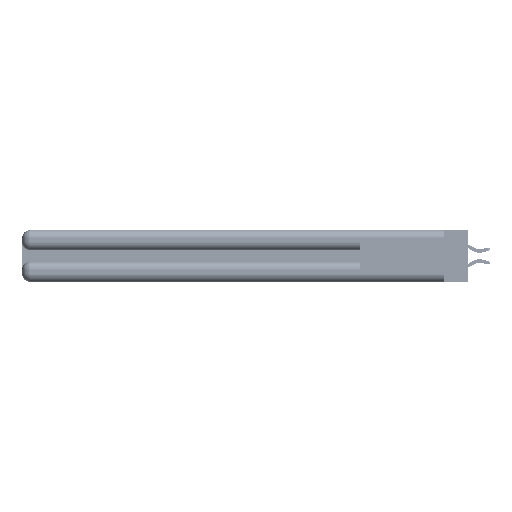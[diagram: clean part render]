
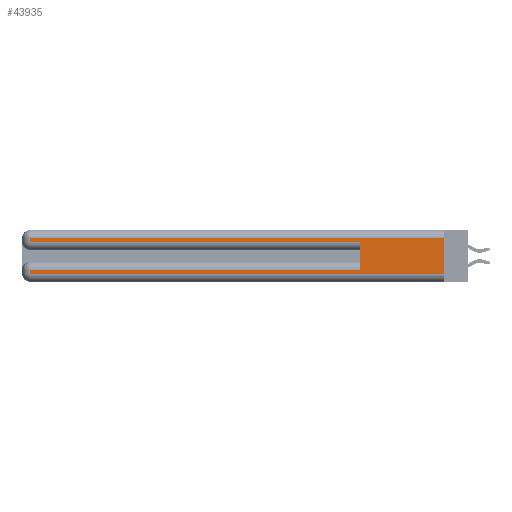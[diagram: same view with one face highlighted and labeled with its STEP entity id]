
A CAD part, left-side view. The second image highlights one B-rep face of the part: STEP entity #43935.
In plain terms, the highlighted planar face has unit normal (-1, 0, 0).
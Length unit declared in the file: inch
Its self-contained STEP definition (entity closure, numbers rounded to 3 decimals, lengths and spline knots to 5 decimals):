
#156 = CARTESIAN_POINT ( 'NONE',  ( 0., 0., 0.37 ) ) ;
#1914 = EDGE_CURVE ( 'NONE', #38945, #14404, #46046, .T. ) ;
#2449 = ORIENTED_EDGE ( 'NONE', *, *, #48243, .T. ) ;
#3163 = VECTOR ( 'NONE', #41741, 39.37008 ) ;
#4113 = EDGE_CURVE ( 'NONE', #38985, #38945, #40312, .T. ) ;
#4177 = DIRECTION ( 'NONE',  ( 0., 0., -1. ) ) ;
#4496 = CARTESIAN_POINT ( 'NONE',  ( 0., 2.94, 0.06 ) ) ;
#4733 = CARTESIAN_POINT ( 'NONE',  ( 0., 0., 0.285 ) ) ;
#7705 = VECTOR ( 'NONE', #36202, 39.37008 ) ;
#8487 = LINE ( 'NONE', #11808, #47719 ) ;
#9057 = EDGE_CURVE ( 'NONE', #34411, #14404, #26335, .T. ) ;
#10881 = DIRECTION ( 'NONE',  ( 0., 0., -1. ) ) ;
#11180 = CARTESIAN_POINT ( 'NONE',  ( 0., 2.94, 0.37 ) ) ;
#11744 = EDGE_CURVE ( 'NONE', #30185, #33494, #34601, .T. ) ;
#11808 = CARTESIAN_POINT ( 'NONE',  ( 0., 0.6, 0.145 ) ) ;
#11882 = ORIENTED_EDGE ( 'NONE', *, *, #9057, .F. ) ;
#12680 = CARTESIAN_POINT ( 'NONE',  ( 0., 2.94, 0.085 ) ) ;
#13272 = CARTESIAN_POINT ( 'NONE',  ( 0., 0., 0.06 ) ) ;
#14369 = CARTESIAN_POINT ( 'NONE',  ( 0., 0., 0.31 ) ) ;
#14404 = VERTEX_POINT ( 'NONE', #14673 ) ;
#14500 = CARTESIAN_POINT ( 'NONE',  ( 0., 2.94, 0.285 ) ) ;
#14673 = CARTESIAN_POINT ( 'NONE',  ( 0., 0., 0.06 ) ) ;
#15150 = DIRECTION ( 'NONE',  ( 0., 0., -1. ) ) ;
#15244 = VECTOR ( 'NONE', #17268, 39.37008 ) ;
#17268 = DIRECTION ( 'NONE',  ( 0., 1., 0. ) ) ;
#18251 = LINE ( 'NONE', #4733, #7705 ) ;
#19418 = EDGE_CURVE ( 'NONE', #33494, #39468, #18251, .T. ) ;
#19722 = CARTESIAN_POINT ( 'NONE',  ( 0., 0.6, 0.085 ) ) ;
#21743 = ORIENTED_EDGE ( 'NONE', *, *, #19418, .T. ) ;
#25411 = ORIENTED_EDGE ( 'NONE', *, *, #4113, .T. ) ;
#26335 = LINE ( 'NONE', #30435, #44681 ) ;
#26481 = VECTOR ( 'NONE', #40627, 39.37008 ) ;
#27783 = DIRECTION ( 'NONE',  ( 1., 0., 0. ) ) ;
#28116 = LINE ( 'NONE', #28885, #15244 ) ;
#28414 = EDGE_LOOP ( 'NONE', ( #11882, #2449, #42818, #21743, #45611, #45478, #25411, #43830 ) ) ;
#28479 = EDGE_CURVE ( 'NONE', #30929, #38985, #28116, .T. ) ;
#28885 = CARTESIAN_POINT ( 'NONE',  ( 0., 0., 0.085 ) ) ;
#30185 = VERTEX_POINT ( 'NONE', #39277 ) ;
#30435 = CARTESIAN_POINT ( 'NONE',  ( 0., 0., 0.37 ) ) ;
#30929 = VERTEX_POINT ( 'NONE', #19722 ) ;
#33494 = VERTEX_POINT ( 'NONE', #14500 ) ;
#34411 = VERTEX_POINT ( 'NONE', #36673 ) ;
#34601 = LINE ( 'NONE', #37798, #3163 ) ;
#34914 = EDGE_CURVE ( 'NONE', #30929, #39468, #8487, .T. ) ;
#35256 = DIRECTION ( 'NONE',  ( 0., 0., 1. ) ) ;
#35485 = PLANE ( 'NONE',  #50520 ) ;
#36202 = DIRECTION ( 'NONE',  ( 0., -1., 0. ) ) ;
#36673 = CARTESIAN_POINT ( 'NONE',  ( 0., 0., 0.31 ) ) ;
#37128 = FACE_OUTER_BOUND ( 'NONE', #28414, .T. ) ;
#37798 = CARTESIAN_POINT ( 'NONE',  ( 0., 2.94, 0.37 ) ) ;
#37814 = DIRECTION ( 'NONE',  ( 0., 1., 0. ) ) ;
#38945 = VERTEX_POINT ( 'NONE', #4496 ) ;
#38985 = VERTEX_POINT ( 'NONE', #12680 ) ;
#39277 = CARTESIAN_POINT ( 'NONE',  ( 0., 2.94, 0.31 ) ) ;
#39468 = VERTEX_POINT ( 'NONE', #42569 ) ;
#40312 = LINE ( 'NONE', #11180, #42778 ) ;
#40627 = DIRECTION ( 'NONE',  ( 0., -1., 0. ) ) ;
#41741 = DIRECTION ( 'NONE',  ( 0., 0., -1. ) ) ;
#42569 = CARTESIAN_POINT ( 'NONE',  ( 0., 0.6, 0.285 ) ) ;
#42778 = VECTOR ( 'NONE', #15150, 39.37008 ) ;
#42818 = ORIENTED_EDGE ( 'NONE', *, *, #11744, .T. ) ;
#42894 = VECTOR ( 'NONE', #37814, 39.37008 ) ;
#43830 = ORIENTED_EDGE ( 'NONE', *, *, #1914, .T. ) ;
#43935 = ADVANCED_FACE ( 'NONE', ( #37128 ), #35485, .F. ) ;
#44681 = VECTOR ( 'NONE', #10881, 39.37008 ) ;
#45333 = LINE ( 'NONE', #14369, #42894 ) ;
#45478 = ORIENTED_EDGE ( 'NONE', *, *, #28479, .T. ) ;
#45611 = ORIENTED_EDGE ( 'NONE', *, *, #34914, .F. ) ;
#46046 = LINE ( 'NONE', #13272, #26481 ) ;
#47719 = VECTOR ( 'NONE', #35256, 39.37008 ) ;
#48243 = EDGE_CURVE ( 'NONE', #34411, #30185, #45333, .T. ) ;
#50520 = AXIS2_PLACEMENT_3D ( 'NONE', #156, #27783, #4177 ) ;
